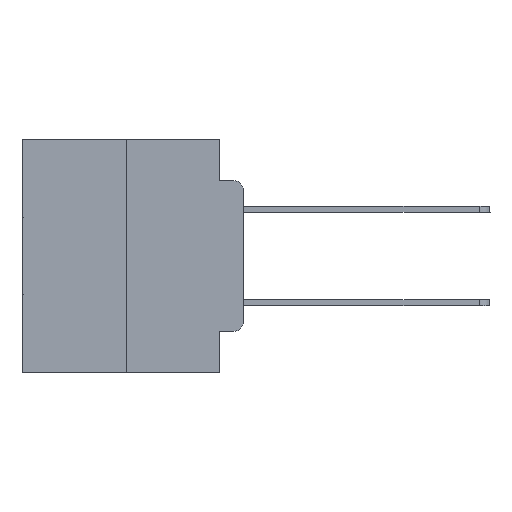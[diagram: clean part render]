
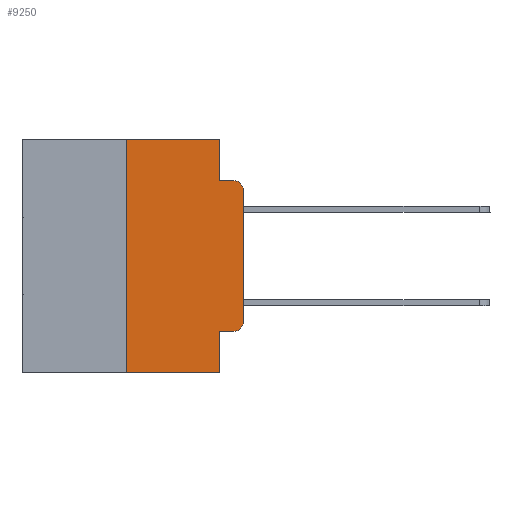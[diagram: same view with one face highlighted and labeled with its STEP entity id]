
A CAD part, left-side view. The second image highlights one B-rep face of the part: STEP entity #9250.
In plain terms, the highlighted planar face has unit normal (-1, 0, 0).
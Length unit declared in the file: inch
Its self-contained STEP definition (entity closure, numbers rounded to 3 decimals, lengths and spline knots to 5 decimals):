
#919 = VERTEX_POINT ( 'NONE', #2662 ) ;
#955 = CARTESIAN_POINT ( 'NONE',  ( 0., 0., -0.1085 ) ) ;
#1118 = EDGE_CURVE ( 'NONE', #26984, #919, #19530, .T. ) ;
#2257 = ORIENTED_EDGE ( 'NONE', *, *, #20684, .T. ) ;
#2421 = AXIS2_PLACEMENT_3D ( 'NONE', #5808, #20130, #6750 ) ;
#2662 = CARTESIAN_POINT ( 'NONE',  ( 0., 0.051, -0.5 ) ) ;
#2839 = DIRECTION ( 'NONE',  ( 0., -1., 0. ) ) ;
#2863 = DIRECTION ( 'NONE',  ( 0., -1., 0. ) ) ;
#3146 = ORIENTED_EDGE ( 'NONE', *, *, #23786, .F. ) ;
#4280 = ORIENTED_EDGE ( 'NONE', *, *, #27695, .F. ) ;
#4425 = VECTOR ( 'NONE', #2863, 39.37008 ) ;
#4609 = CARTESIAN_POINT ( 'NONE',  ( 0., 0.051, 0. ) ) ;
#5499 = VERTEX_POINT ( 'NONE', #23276 ) ;
#5671 = FACE_OUTER_BOUND ( 'NONE', #22163, .T. ) ;
#5762 = DIRECTION ( 'NONE',  ( 0., 0., -1. ) ) ;
#5808 = CARTESIAN_POINT ( 'NONE',  ( 0., 0.02, -0.3915 ) ) ;
#6750 = DIRECTION ( 'NONE',  ( 0., 0., -1. ) ) ;
#6815 = VECTOR ( 'NONE', #2839, 39.37008 ) ;
#7286 = VECTOR ( 'NONE', #5762, 39.37008 ) ;
#7796 = CARTESIAN_POINT ( 'NONE',  ( 0., 0.02, -0.0885 ) ) ;
#7816 = CARTESIAN_POINT ( 'NONE',  ( 0., 0.051, -0.0885 ) ) ;
#8188 = AXIS2_PLACEMENT_3D ( 'NONE', #13545, #30388, #16095 ) ;
#9158 = ORIENTED_EDGE ( 'NONE', *, *, #15429, .T. ) ;
#9225 = EDGE_CURVE ( 'NONE', #20576, #9757, #24951, .T. ) ;
#9250 = ADVANCED_FACE ( 'NONE', ( #5671 ), #12697, .F. ) ;
#9342 = EDGE_CURVE ( 'NONE', #30436, #919, #19391, .T. ) ;
#9439 = LINE ( 'NONE', #11348, #15386 ) ;
#9757 = VERTEX_POINT ( 'NONE', #7796 ) ;
#10506 = DIRECTION ( 'NONE',  ( 0., -1., 0. ) ) ;
#10568 = CIRCLE ( 'NONE', #8188, 0.02 ) ;
#11348 = CARTESIAN_POINT ( 'NONE',  ( 0., 0.25, 0. ) ) ;
#11571 = VERTEX_POINT ( 'NONE', #30802 ) ;
#11705 = ORIENTED_EDGE ( 'NONE', *, *, #19594, .F. ) ;
#12435 = CARTESIAN_POINT ( 'NONE',  ( 0., 0., 0. ) ) ;
#12495 = CARTESIAN_POINT ( 'NONE',  ( 0., 0.02, -0.4115 ) ) ;
#12697 = PLANE ( 'NONE',  #14424 ) ;
#13229 = CARTESIAN_POINT ( 'NONE',  ( 0., 0.473, 0. ) ) ;
#13545 = CARTESIAN_POINT ( 'NONE',  ( 0., 0.02, -0.1085 ) ) ;
#13842 = DIRECTION ( 'NONE',  ( 0., -1., 0. ) ) ;
#14424 = AXIS2_PLACEMENT_3D ( 'NONE', #13229, #22438, #22322 ) ;
#15284 = CIRCLE ( 'NONE', #2421, 0.02 ) ;
#15386 = VECTOR ( 'NONE', #27971, 39.37008 ) ;
#15429 = EDGE_CURVE ( 'NONE', #29715, #5499, #15284, .T. ) ;
#16095 = DIRECTION ( 'NONE',  ( 0., 0., -1. ) ) ;
#16653 = ORIENTED_EDGE ( 'NONE', *, *, #26755, .T. ) ;
#18033 = VECTOR ( 'NONE', #13842, 39.37008 ) ;
#18248 = ORIENTED_EDGE ( 'NONE', *, *, #26762, .T. ) ;
#18291 = DIRECTION ( 'NONE',  ( 0., 0., -1. ) ) ;
#18438 = ORIENTED_EDGE ( 'NONE', *, *, #9342, .T. ) ;
#18681 = LINE ( 'NONE', #4609, #26098 ) ;
#19220 = VECTOR ( 'NONE', #28749, 39.37008 ) ;
#19391 = LINE ( 'NONE', #24692, #24924 ) ;
#19530 = LINE ( 'NONE', #22267, #7286 ) ;
#19578 = LINE ( 'NONE', #12435, #19220 ) ;
#19594 = EDGE_CURVE ( 'NONE', #30436, #11571, #9439, .T. ) ;
#20130 = DIRECTION ( 'NONE',  ( -1., 0., 0. ) ) ;
#20439 = CARTESIAN_POINT ( 'NONE',  ( 0., 0.25, -0.5 ) ) ;
#20576 = VERTEX_POINT ( 'NONE', #21966 ) ;
#20684 = EDGE_CURVE ( 'NONE', #5499, #29218, #19578, .T. ) ;
#21138 = LINE ( 'NONE', #29042, #4425 ) ;
#21270 = CARTESIAN_POINT ( 'NONE',  ( 0., 0.051, -0.4115 ) ) ;
#21966 = CARTESIAN_POINT ( 'NONE',  ( 0., 0.051, -0.0885 ) ) ;
#22121 = CARTESIAN_POINT ( 'NONE',  ( 0., 0.051, 0. ) ) ;
#22163 = EDGE_LOOP ( 'NONE', ( #2257, #18248, #27174, #4280, #3146, #11705, #18438, #24300, #16653, #9158 ) ) ;
#22267 = CARTESIAN_POINT ( 'NONE',  ( 0., 0.051, 0. ) ) ;
#22322 = DIRECTION ( 'NONE',  ( 0., 0., -1. ) ) ;
#22438 = DIRECTION ( 'NONE',  ( 1., 0., 0. ) ) ;
#23276 = CARTESIAN_POINT ( 'NONE',  ( 0., 0., -0.3915 ) ) ;
#23786 = EDGE_CURVE ( 'NONE', #11571, #27849, #21138, .T. ) ;
#23910 = LINE ( 'NONE', #30171, #18033 ) ;
#24300 = ORIENTED_EDGE ( 'NONE', *, *, #1118, .F. ) ;
#24692 = CARTESIAN_POINT ( 'NONE',  ( 0., 0.473, -0.5 ) ) ;
#24924 = VECTOR ( 'NONE', #10506, 39.37008 ) ;
#24951 = LINE ( 'NONE', #7816, #6815 ) ;
#26098 = VECTOR ( 'NONE', #18291, 39.37008 ) ;
#26755 = EDGE_CURVE ( 'NONE', #26984, #29715, #23910, .T. ) ;
#26762 = EDGE_CURVE ( 'NONE', #29218, #9757, #10568, .T. ) ;
#26984 = VERTEX_POINT ( 'NONE', #21270 ) ;
#27174 = ORIENTED_EDGE ( 'NONE', *, *, #9225, .F. ) ;
#27695 = EDGE_CURVE ( 'NONE', #27849, #20576, #18681, .T. ) ;
#27849 = VERTEX_POINT ( 'NONE', #22121 ) ;
#27971 = DIRECTION ( 'NONE',  ( 0., 0., 1. ) ) ;
#28749 = DIRECTION ( 'NONE',  ( 0., 0., 1. ) ) ;
#29042 = CARTESIAN_POINT ( 'NONE',  ( 0., 0.473, 0. ) ) ;
#29218 = VERTEX_POINT ( 'NONE', #955 ) ;
#29715 = VERTEX_POINT ( 'NONE', #12495 ) ;
#30171 = CARTESIAN_POINT ( 'NONE',  ( 0., 0.051, -0.4115 ) ) ;
#30388 = DIRECTION ( 'NONE',  ( -1., 0., 0. ) ) ;
#30436 = VERTEX_POINT ( 'NONE', #20439 ) ;
#30802 = CARTESIAN_POINT ( 'NONE',  ( 0., 0.25, 0. ) ) ;
